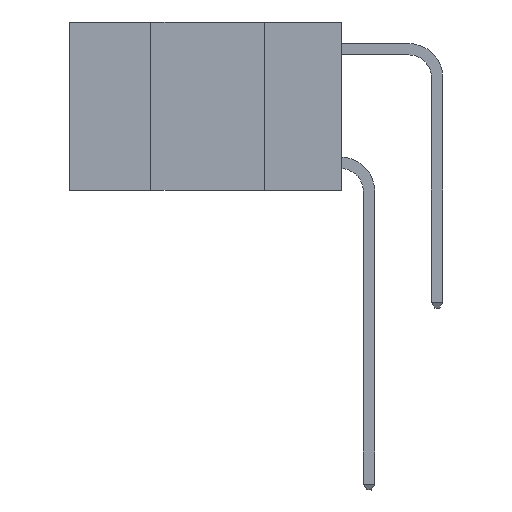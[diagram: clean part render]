
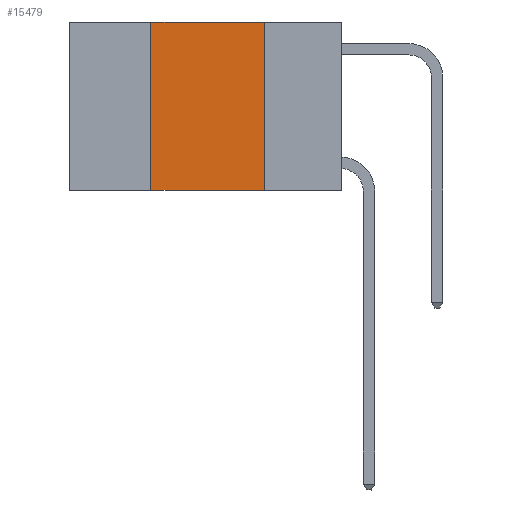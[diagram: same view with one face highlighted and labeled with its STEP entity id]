
A CAD part, left-side view. The second image highlights one B-rep face of the part: STEP entity #15479.
In plain terms, the highlighted planar face has unit normal (-1, 0, 0).
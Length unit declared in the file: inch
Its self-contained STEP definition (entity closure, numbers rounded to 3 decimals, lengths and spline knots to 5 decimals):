
#9 = CARTESIAN_POINT ( 'NONE',  ( 0., 0.42, 0. ) ) ;
#1057 = AXIS2_PLACEMENT_3D ( 'NONE', #14106, #15795, #5619 ) ;
#1551 = LINE ( 'NONE', #17868, #10669 ) ;
#1582 = EDGE_CURVE ( 'NONE', #13420, #2667, #16340, .T. ) ;
#2667 = VERTEX_POINT ( 'NONE', #5707 ) ;
#3873 = PLANE ( 'NONE',  #1057 ) ;
#5307 = FACE_OUTER_BOUND ( 'NONE', #20263, .T. ) ;
#5396 = DIRECTION ( 'NONE',  ( 0., -1., 0. ) ) ;
#5619 = DIRECTION ( 'NONE',  ( 0., 0., -1. ) ) ;
#5707 = CARTESIAN_POINT ( 'NONE',  ( 0., 0.17, 0. ) ) ;
#6138 = EDGE_CURVE ( 'NONE', #6524, #16987, #18200, .T. ) ;
#6524 = VERTEX_POINT ( 'NONE', #10734 ) ;
#6623 = ORIENTED_EDGE ( 'NONE', *, *, #20290, .F. ) ;
#6716 = LINE ( 'NONE', #14013, #15235 ) ;
#7256 = DIRECTION ( 'NONE',  ( 0., 0., -1. ) ) ;
#7407 = CARTESIAN_POINT ( 'NONE',  ( 0., 0.17, -0.37 ) ) ;
#7667 = DIRECTION ( 'NONE',  ( 0., 0., 1. ) ) ;
#10669 = VECTOR ( 'NONE', #7667, 39.37008 ) ;
#10734 = CARTESIAN_POINT ( 'NONE',  ( 0., 0.42, -0.37 ) ) ;
#11681 = ORIENTED_EDGE ( 'NONE', *, *, #6138, .T. ) ;
#11945 = ORIENTED_EDGE ( 'NONE', *, *, #14143, .F. ) ;
#13420 = VERTEX_POINT ( 'NONE', #9 ) ;
#13729 = VECTOR ( 'NONE', #5396, 39.37008 ) ;
#14013 = CARTESIAN_POINT ( 'NONE',  ( 0., 0.17, 0. ) ) ;
#14106 = CARTESIAN_POINT ( 'NONE',  ( 0., 0.6, 0. ) ) ;
#14143 = EDGE_CURVE ( 'NONE', #2667, #16987, #6716, .T. ) ;
#14619 = ORIENTED_EDGE ( 'NONE', *, *, #1582, .F. ) ;
#15235 = VECTOR ( 'NONE', #7256, 39.37008 ) ;
#15479 = ADVANCED_FACE ( 'NONE', ( #5307 ), #3873, .F. ) ;
#15795 = DIRECTION ( 'NONE',  ( 1., 0., 0. ) ) ;
#15819 = VECTOR ( 'NONE', #21552, 39.37008 ) ;
#16340 = LINE ( 'NONE', #21448, #15819 ) ;
#16987 = VERTEX_POINT ( 'NONE', #7407 ) ;
#17868 = CARTESIAN_POINT ( 'NONE',  ( 0., 0.42, 0. ) ) ;
#18200 = LINE ( 'NONE', #20694, #13729 ) ;
#20263 = EDGE_LOOP ( 'NONE', ( #11945, #14619, #6623, #11681 ) ) ;
#20290 = EDGE_CURVE ( 'NONE', #6524, #13420, #1551, .T. ) ;
#20694 = CARTESIAN_POINT ( 'NONE',  ( 0., 0.6, -0.37 ) ) ;
#21448 = CARTESIAN_POINT ( 'NONE',  ( 0., 0.6, 0. ) ) ;
#21552 = DIRECTION ( 'NONE',  ( 0., -1., 0. ) ) ;
